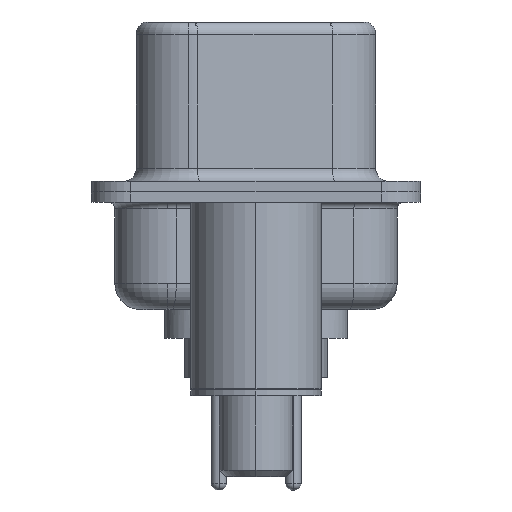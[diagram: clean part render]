
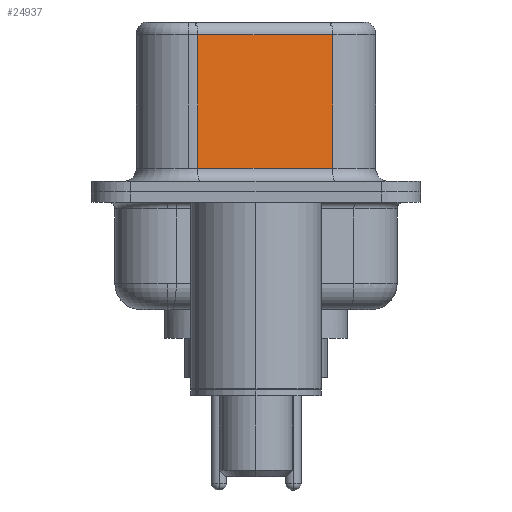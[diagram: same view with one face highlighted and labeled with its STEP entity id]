
A CAD part, left-side view. The second image highlights one B-rep face of the part: STEP entity #24937.
In plain terms, the highlighted planar face has unit normal (-0.985, -0.174, 0).
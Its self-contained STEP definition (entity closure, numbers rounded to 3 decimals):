
#114 = CARTESIAN_POINT ( 'NONE',  ( 4.58, -2.927, 6.52 ) ) ;
#476 = ORIENTED_EDGE ( 'NONE', *, *, #18559, .T. ) ;
#804 = CARTESIAN_POINT ( 'NONE',  ( 4.58, -2.927, 6.02 ) ) ;
#1330 = CARTESIAN_POINT ( 'NONE',  ( 3.67, 2.233, 6.02 ) ) ;
#2479 = EDGE_CURVE ( 'NONE', #23137, #2985, #20443, .T. ) ;
#2985 = VERTEX_POINT ( 'NONE', #21686 ) ;
#3211 = CARTESIAN_POINT ( 'NONE',  ( 3.67, 2.233, 0.9 ) ) ;
#4558 = ORIENTED_EDGE ( 'NONE', *, *, #2479, .T. ) ;
#4676 = DIRECTION ( 'NONE',  ( 0.985, 0.174, 0. ) ) ;
#6000 = EDGE_CURVE ( 'NONE', #8490, #2985, #13733, .T. ) ;
#7009 = DIRECTION ( 'NONE',  ( -0.174, 0.985, 0. ) ) ;
#7065 = DIRECTION ( 'NONE',  ( 0.174, -0.985, 0. ) ) ;
#8490 = VERTEX_POINT ( 'NONE', #27286 ) ;
#8823 = VECTOR ( 'NONE', #27061, 1000. ) ;
#8827 = CARTESIAN_POINT ( 'NONE',  ( 4.58, -2.927, 6.52 ) ) ;
#9578 = VECTOR ( 'NONE', #23485, 1000. ) ;
#9823 = VECTOR ( 'NONE', #7065, 1000. ) ;
#10135 = FACE_OUTER_BOUND ( 'NONE', #22013, .T. ) ;
#11242 = EDGE_CURVE ( 'NONE', #14401, #23137, #20890, .T. ) ;
#12857 = CARTESIAN_POINT ( 'NONE',  ( 3.67, 2.233, 6.52 ) ) ;
#13049 = PLANE ( 'NONE',  #19068 ) ;
#13733 = LINE ( 'NONE', #114, #8823 ) ;
#13864 = CARTESIAN_POINT ( 'NONE',  ( 4.58, -2.927, 0.9 ) ) ;
#14401 = VERTEX_POINT ( 'NONE', #1330 ) ;
#16521 = ORIENTED_EDGE ( 'NONE', *, *, #6000, .F. ) ;
#18559 = EDGE_CURVE ( 'NONE', #8490, #14401, #20326, .T. ) ;
#19068 = AXIS2_PLACEMENT_3D ( 'NONE', #8827, #4676, #19470 ) ;
#19470 = DIRECTION ( 'NONE',  ( -0.174, 0.985, 0. ) ) ;
#19646 = VECTOR ( 'NONE', #7009, 1000. ) ;
#20326 = LINE ( 'NONE', #804, #19646 ) ;
#20443 = LINE ( 'NONE', #13864, #9823 ) ;
#20890 = LINE ( 'NONE', #12857, #9578 ) ;
#21686 = CARTESIAN_POINT ( 'NONE',  ( 4.58, -2.927, 0.9 ) ) ;
#22013 = EDGE_LOOP ( 'NONE', ( #16521, #476, #22615, #4558 ) ) ;
#22615 = ORIENTED_EDGE ( 'NONE', *, *, #11242, .T. ) ;
#23137 = VERTEX_POINT ( 'NONE', #3211 ) ;
#23485 = DIRECTION ( 'NONE',  ( 0., 0., -1. ) ) ;
#24937 = ADVANCED_FACE ( 'NONE', ( #10135 ), #13049, .F. ) ;
#27061 = DIRECTION ( 'NONE',  ( 0., 0., -1. ) ) ;
#27286 = CARTESIAN_POINT ( 'NONE',  ( 4.58, -2.927, 6.02 ) ) ;
